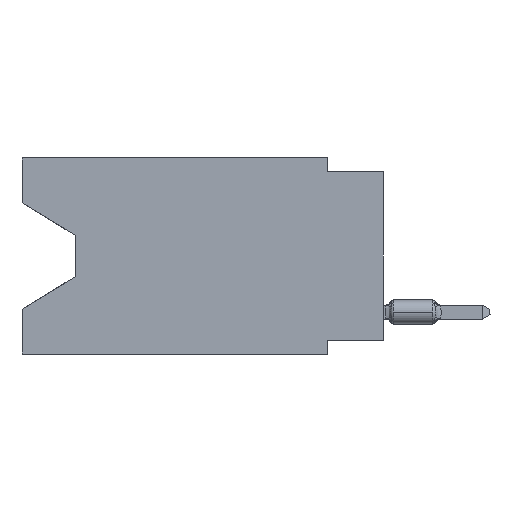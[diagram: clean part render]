
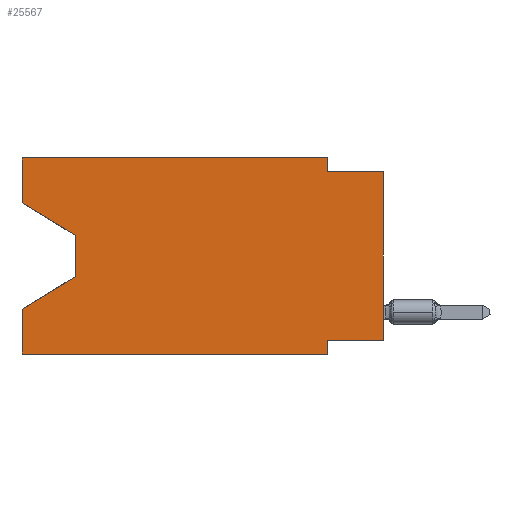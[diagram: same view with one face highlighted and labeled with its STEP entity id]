
A CAD part, left-side view. The second image highlights one B-rep face of the part: STEP entity #25567.
In plain terms, the highlighted planar face has unit normal (-1, 0, 0).
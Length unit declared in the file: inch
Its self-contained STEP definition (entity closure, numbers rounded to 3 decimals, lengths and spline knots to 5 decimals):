
#529 = CARTESIAN_POINT ( 'NONE',  ( 0., 0., -0.325 ) ) ;
#735 = CARTESIAN_POINT ( 'NONE',  ( 0., 0.645, -0.35 ) ) ;
#997 = DIRECTION ( 'NONE',  ( 0., 0., -1. ) ) ;
#1016 = EDGE_CURVE ( 'NONE', #15420, #2341, #34021, .T. ) ;
#1786 = ORIENTED_EDGE ( 'NONE', *, *, #16227, .F. ) ;
#1955 = DIRECTION ( 'NONE',  ( 0., 1., 0. ) ) ;
#2341 = VERTEX_POINT ( 'NONE', #6181 ) ;
#2427 = CARTESIAN_POINT ( 'NONE',  ( 0., 0.645, 0. ) ) ;
#2688 = VECTOR ( 'NONE', #9881, 39.37008 ) ;
#2724 = CARTESIAN_POINT ( 'NONE',  ( 0., 0.645, 0. ) ) ;
#3183 = ORIENTED_EDGE ( 'NONE', *, *, #36033, .T. ) ;
#3270 = ORIENTED_EDGE ( 'NONE', *, *, #22229, .T. ) ;
#3683 = LINE ( 'NONE', #6779, #13491 ) ;
#5614 = ORIENTED_EDGE ( 'NONE', *, *, #13958, .F. ) ;
#5837 = CARTESIAN_POINT ( 'NONE',  ( 0., 0.55, -0.212 ) ) ;
#5997 = LINE ( 'NONE', #17772, #6927 ) ;
#6039 = CARTESIAN_POINT ( 'NONE',  ( 0., 0.55, -0.212 ) ) ;
#6181 = CARTESIAN_POINT ( 'NONE',  ( 0., 0., -0.025 ) ) ;
#6482 = ORIENTED_EDGE ( 'NONE', *, *, #24849, .T. ) ;
#6750 = DIRECTION ( 'NONE',  ( 0., -1., 0. ) ) ;
#6779 = CARTESIAN_POINT ( 'NONE',  ( 0., 0.1, -0.35 ) ) ;
#6927 = VECTOR ( 'NONE', #9453, 39.37008 ) ;
#7813 = EDGE_CURVE ( 'NONE', #21274, #32039, #8169, .T. ) ;
#7892 = ORIENTED_EDGE ( 'NONE', *, *, #36312, .T. ) ;
#7917 = VERTEX_POINT ( 'NONE', #5837 ) ;
#8000 = CARTESIAN_POINT ( 'NONE',  ( 0., 0.1, 0. ) ) ;
#8042 = FACE_OUTER_BOUND ( 'NONE', #20713, .T. ) ;
#8169 = LINE ( 'NONE', #31746, #29137 ) ;
#8435 = CARTESIAN_POINT ( 'NONE',  ( 0., 0.645, 0. ) ) ;
#8843 = VERTEX_POINT ( 'NONE', #21904 ) ;
#9005 = EDGE_CURVE ( 'NONE', #7917, #29574, #23623, .T. ) ;
#9247 = CARTESIAN_POINT ( 'NONE',  ( 0., 0.1, -0.35 ) ) ;
#9453 = DIRECTION ( 'NONE',  ( 0., 0., 1. ) ) ;
#9681 = DIRECTION ( 'NONE',  ( 0., 0., -1. ) ) ;
#9881 = DIRECTION ( 'NONE',  ( 0., -1., 0. ) ) ;
#9889 = VERTEX_POINT ( 'NONE', #12008 ) ;
#10905 = LINE ( 'NONE', #23272, #32934 ) ;
#10990 = LINE ( 'NONE', #28770, #36548 ) ;
#11092 = DIRECTION ( 'NONE',  ( 0., 0., -1. ) ) ;
#11249 = DIRECTION ( 'NONE',  ( 0., -1., 0. ) ) ;
#11519 = DIRECTION ( 'NONE',  ( 0., 0., -1. ) ) ;
#11719 = DIRECTION ( 'NONE',  ( 0., 0., 1. ) ) ;
#12008 = CARTESIAN_POINT ( 'NONE',  ( 0., 0.645, 0. ) ) ;
#12615 = CARTESIAN_POINT ( 'NONE',  ( 0., 0.55, -0.138 ) ) ;
#12946 = CARTESIAN_POINT ( 'NONE',  ( 0., 0.1, 0. ) ) ;
#13491 = VECTOR ( 'NONE', #9681, 39.37008 ) ;
#13958 = EDGE_CURVE ( 'NONE', #31752, #15420, #17255, .T. ) ;
#13965 = EDGE_CURVE ( 'NONE', #17164, #9889, #10905, .T. ) ;
#15420 = VERTEX_POINT ( 'NONE', #31492 ) ;
#15520 = LINE ( 'NONE', #12615, #16592 ) ;
#16227 = EDGE_CURVE ( 'NONE', #9889, #31752, #22651, .T. ) ;
#16446 = EDGE_CURVE ( 'NONE', #32039, #22392, #3683, .T. ) ;
#16592 = VECTOR ( 'NONE', #997, 39.37008 ) ;
#17146 = ORIENTED_EDGE ( 'NONE', *, *, #1016, .F. ) ;
#17164 = VERTEX_POINT ( 'NONE', #19263 ) ;
#17255 = LINE ( 'NONE', #8000, #17477 ) ;
#17477 = VECTOR ( 'NONE', #11092, 39.37008 ) ;
#17772 = CARTESIAN_POINT ( 'NONE',  ( 0., 0., 0. ) ) ;
#17902 = VECTOR ( 'NONE', #29613, 39.37008 ) ;
#18725 = EDGE_CURVE ( 'NONE', #32488, #29574, #34345, .T. ) ;
#18900 = ORIENTED_EDGE ( 'NONE', *, *, #18725, .F. ) ;
#19263 = CARTESIAN_POINT ( 'NONE',  ( 0., 0.645, -0.08025 ) ) ;
#19327 = CARTESIAN_POINT ( 'NONE',  ( 0., 0., -0.025 ) ) ;
#19704 = CARTESIAN_POINT ( 'NONE',  ( 0., 0.645, -0.26975 ) ) ;
#20713 = EDGE_LOOP ( 'NONE', ( #7892, #3270, #34991, #18900, #6482, #30241, #27301, #3183, #17146, #5614, #1786, #35017 ) ) ;
#21274 = VERTEX_POINT ( 'NONE', #529 ) ;
#21904 = CARTESIAN_POINT ( 'NONE',  ( 0., 0.55, -0.138 ) ) ;
#22229 = EDGE_CURVE ( 'NONE', #8843, #7917, #15520, .T. ) ;
#22392 = VERTEX_POINT ( 'NONE', #9247 ) ;
#22586 = DIRECTION ( 'NONE',  ( 0., -0.855, -0.519 ) ) ;
#22651 = LINE ( 'NONE', #2724, #25226 ) ;
#23272 = CARTESIAN_POINT ( 'NONE',  ( 0., 0.645, 0. ) ) ;
#23623 = LINE ( 'NONE', #6039, #17902 ) ;
#24849 = EDGE_CURVE ( 'NONE', #32488, #22392, #27611, .T. ) ;
#25226 = VECTOR ( 'NONE', #11249, 39.37008 ) ;
#25567 = ADVANCED_FACE ( 'NONE', ( #8042 ), #34514, .F. ) ;
#26484 = VECTOR ( 'NONE', #6750, 39.37008 ) ;
#26516 = AXIS2_PLACEMENT_3D ( 'NONE', #8435, #28905, #11519 ) ;
#27301 = ORIENTED_EDGE ( 'NONE', *, *, #7813, .F. ) ;
#27611 = LINE ( 'NONE', #735, #26484 ) ;
#28770 = CARTESIAN_POINT ( 'NONE',  ( 0., 0.645, -0.08025 ) ) ;
#28905 = DIRECTION ( 'NONE',  ( 1., 0., 0. ) ) ;
#29137 = VECTOR ( 'NONE', #1955, 39.37008 ) ;
#29574 = VERTEX_POINT ( 'NONE', #19704 ) ;
#29613 = DIRECTION ( 'NONE',  ( 0., 0.855, -0.519 ) ) ;
#30241 = ORIENTED_EDGE ( 'NONE', *, *, #16446, .F. ) ;
#30810 = CARTESIAN_POINT ( 'NONE',  ( 0., 0.645, -0.35 ) ) ;
#30860 = CARTESIAN_POINT ( 'NONE',  ( 0., 0.1, -0.325 ) ) ;
#31089 = VECTOR ( 'NONE', #11719, 39.37008 ) ;
#31492 = CARTESIAN_POINT ( 'NONE',  ( 0., 0.1, -0.025 ) ) ;
#31746 = CARTESIAN_POINT ( 'NONE',  ( 0., 0., -0.325 ) ) ;
#31752 = VERTEX_POINT ( 'NONE', #12946 ) ;
#32039 = VERTEX_POINT ( 'NONE', #30860 ) ;
#32488 = VERTEX_POINT ( 'NONE', #30810 ) ;
#32934 = VECTOR ( 'NONE', #35049, 39.37008 ) ;
#34021 = LINE ( 'NONE', #19327, #2688 ) ;
#34345 = LINE ( 'NONE', #2427, #31089 ) ;
#34514 = PLANE ( 'NONE',  #26516 ) ;
#34991 = ORIENTED_EDGE ( 'NONE', *, *, #9005, .T. ) ;
#35017 = ORIENTED_EDGE ( 'NONE', *, *, #13965, .F. ) ;
#35049 = DIRECTION ( 'NONE',  ( 0., 0., 1. ) ) ;
#36033 = EDGE_CURVE ( 'NONE', #21274, #2341, #5997, .T. ) ;
#36312 = EDGE_CURVE ( 'NONE', #17164, #8843, #10990, .T. ) ;
#36548 = VECTOR ( 'NONE', #22586, 39.37008 ) ;
